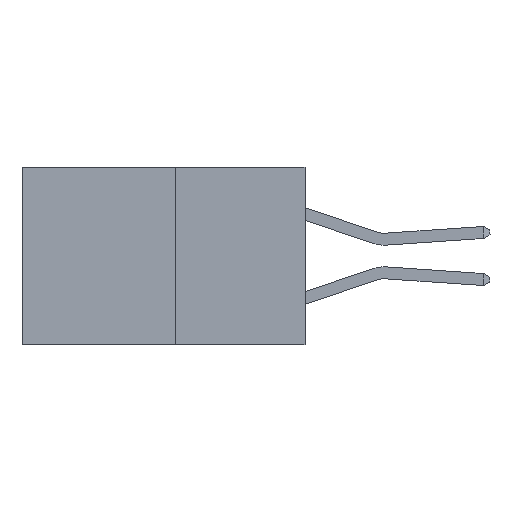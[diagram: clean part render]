
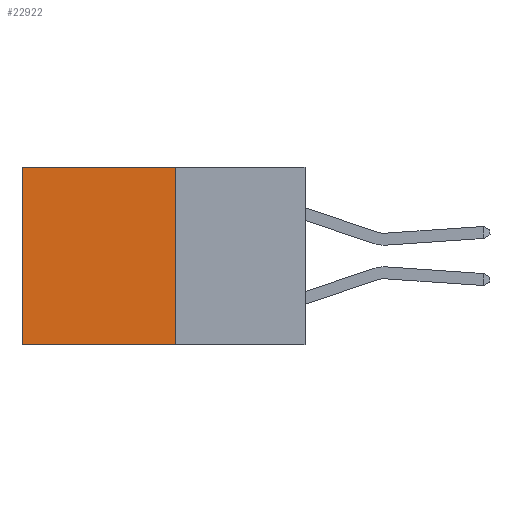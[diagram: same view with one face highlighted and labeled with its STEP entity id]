
A CAD part, left-side view. The second image highlights one B-rep face of the part: STEP entity #22922.
In plain terms, the highlighted planar face has unit normal (-1, 0, 0).
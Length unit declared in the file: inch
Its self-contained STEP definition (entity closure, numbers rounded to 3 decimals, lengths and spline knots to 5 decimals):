
#169 = CARTESIAN_POINT ( 'NONE',  ( 0.277, 0.27, 0. ) ) ;
#400 = VECTOR ( 'NONE', #4829, 39.37008 ) ;
#559 = ORIENTED_EDGE ( 'NONE', *, *, #15749, .F. ) ;
#1229 = LINE ( 'NONE', #10343, #6270 ) ;
#1651 = EDGE_LOOP ( 'NONE', ( #14369, #23241, #559, #7164 ) ) ;
#2181 = PLANE ( 'NONE',  #6388 ) ;
#2337 = VERTEX_POINT ( 'NONE', #12007 ) ;
#4829 = DIRECTION ( 'NONE',  ( 0., 1., 0. ) ) ;
#5164 = LINE ( 'NONE', #6304, #15127 ) ;
#5555 = EDGE_CURVE ( 'NONE', #6931, #17542, #10474, .T. ) ;
#5988 = DIRECTION ( 'NONE',  ( 0., 0., -1. ) ) ;
#6270 = VECTOR ( 'NONE', #21364, 39.37008 ) ;
#6304 = CARTESIAN_POINT ( 'NONE',  ( 0.277, 0.27, -0.37 ) ) ;
#6388 = AXIS2_PLACEMENT_3D ( 'NONE', #15298, #17129, #5988 ) ;
#6931 = VERTEX_POINT ( 'NONE', #22769 ) ;
#7164 = ORIENTED_EDGE ( 'NONE', *, *, #10845, .T. ) ;
#10343 = CARTESIAN_POINT ( 'NONE',  ( 0.277, 0.27, 0. ) ) ;
#10360 = DIRECTION ( 'NONE',  ( 0., 0., -1. ) ) ;
#10474 = LINE ( 'NONE', #21465, #400 ) ;
#10845 = EDGE_CURVE ( 'NONE', #22882, #2337, #1229, .T. ) ;
#12007 = CARTESIAN_POINT ( 'NONE',  ( 0.277, 0.59, 0. ) ) ;
#12219 = LINE ( 'NONE', #21383, #14559 ) ;
#14369 = ORIENTED_EDGE ( 'NONE', *, *, #15289, .T. ) ;
#14559 = VECTOR ( 'NONE', #10360, 39.37008 ) ;
#15127 = VECTOR ( 'NONE', #21134, 39.37008 ) ;
#15289 = EDGE_CURVE ( 'NONE', #2337, #17542, #12219, .T. ) ;
#15298 = CARTESIAN_POINT ( 'NONE',  ( 0.277, 0.27, -0.37 ) ) ;
#15749 = EDGE_CURVE ( 'NONE', #22882, #6931, #5164, .T. ) ;
#17070 = CARTESIAN_POINT ( 'NONE',  ( 0.277, 0.59, -0.37 ) ) ;
#17129 = DIRECTION ( 'NONE',  ( 1., 0., 0. ) ) ;
#17542 = VERTEX_POINT ( 'NONE', #17070 ) ;
#20805 = FACE_OUTER_BOUND ( 'NONE', #1651, .T. ) ;
#21134 = DIRECTION ( 'NONE',  ( 0., 0., -1. ) ) ;
#21364 = DIRECTION ( 'NONE',  ( 0., 1., 0. ) ) ;
#21383 = CARTESIAN_POINT ( 'NONE',  ( 0.277, 0.59, -0.37 ) ) ;
#21465 = CARTESIAN_POINT ( 'NONE',  ( 0.277, 0.27, -0.37 ) ) ;
#22769 = CARTESIAN_POINT ( 'NONE',  ( 0.277, 0.27, -0.37 ) ) ;
#22882 = VERTEX_POINT ( 'NONE', #169 ) ;
#22922 = ADVANCED_FACE ( 'NONE', ( #20805 ), #2181, .F. ) ;
#23241 = ORIENTED_EDGE ( 'NONE', *, *, #5555, .F. ) ;
